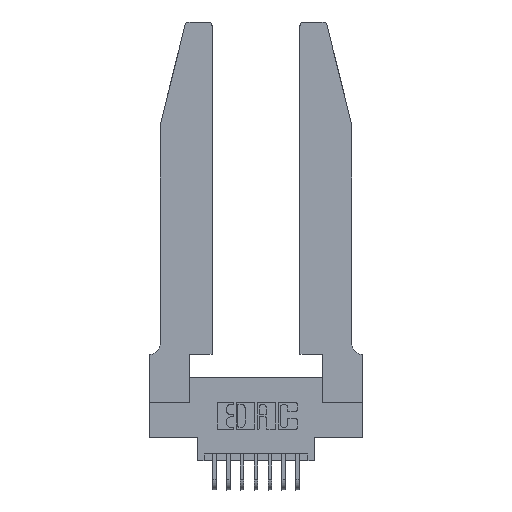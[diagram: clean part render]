
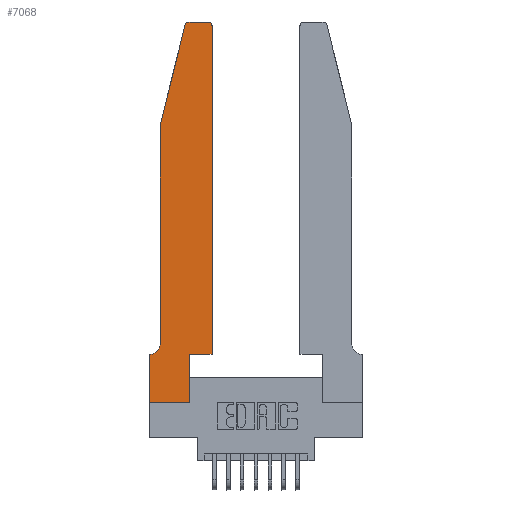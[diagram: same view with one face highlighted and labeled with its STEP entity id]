
A CAD part, top view. The second image highlights one B-rep face of the part: STEP entity #7068.
In plain terms, the highlighted planar face has unit normal (0, 0, 1).
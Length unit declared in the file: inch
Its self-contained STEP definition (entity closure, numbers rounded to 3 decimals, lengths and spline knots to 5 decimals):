
#20 = CARTESIAN_POINT ( 'NONE',  ( 0., 0.35, 0.37 ) ) ;
#129 = VERTEX_POINT ( 'NONE', #14225 ) ;
#232 = VERTEX_POINT ( 'NONE', #20 ) ;
#653 = VECTOR ( 'NONE', #15234, 39.37008 ) ;
#872 = AXIS2_PLACEMENT_3D ( 'NONE', #9520, #1554, #10796 ) ;
#873 = VECTOR ( 'NONE', #11194, 39.37008 ) ;
#876 = VERTEX_POINT ( 'NONE', #8912 ) ;
#995 = VECTOR ( 'NONE', #15243, 39.37008 ) ;
#1045 = VERTEX_POINT ( 'NONE', #2796 ) ;
#1431 = LINE ( 'NONE', #9001, #995 ) ;
#1554 = DIRECTION ( 'NONE',  ( 0., 0., 1. ) ) ;
#1555 = LINE ( 'NONE', #5603, #14964 ) ;
#2014 = CARTESIAN_POINT ( 'NONE',  ( 0.4505, 0.35, 0.37 ) ) ;
#2402 = ORIENTED_EDGE ( 'NONE', *, *, #2558, .T. ) ;
#2558 = EDGE_CURVE ( 'NONE', #129, #6600, #4105, .T. ) ;
#2689 = CARTESIAN_POINT ( 'NONE',  ( 0.2865, 0.35, 0.37 ) ) ;
#2759 = LINE ( 'NONE', #5278, #7181 ) ;
#2796 = CARTESIAN_POINT ( 'NONE',  ( 0.2865, 0., 0.37 ) ) ;
#2841 = VECTOR ( 'NONE', #5559, 39.37008 ) ;
#3032 = VECTOR ( 'NONE', #11817, 39.37008 ) ;
#3412 = AXIS2_PLACEMENT_3D ( 'NONE', #15345, #12888, #5242 ) ;
#4095 = VERTEX_POINT ( 'NONE', #15715 ) ;
#4105 = LINE ( 'NONE', #2014, #873 ) ;
#4113 = CARTESIAN_POINT ( 'NONE',  ( 0.284, 2.72, 0.37 ) ) ;
#4215 = CARTESIAN_POINT ( 'NONE',  ( 0.4505, 0.35, 0.37 ) ) ;
#4342 = VERTEX_POINT ( 'NONE', #11138 ) ;
#5178 = ORIENTED_EDGE ( 'NONE', *, *, #8526, .T. ) ;
#5242 = DIRECTION ( 'NONE',  ( 1., 0., 0. ) ) ;
#5278 = CARTESIAN_POINT ( 'NONE',  ( 0., 0., 0.37 ) ) ;
#5379 = LINE ( 'NONE', #14741, #14745 ) ;
#5454 = DIRECTION ( 'NONE',  ( 1., 0., 0. ) ) ;
#5559 = DIRECTION ( 'NONE',  ( 1., 0., 0. ) ) ;
#5603 = CARTESIAN_POINT ( 'NONE',  ( 0.2605, 2.75, 0.37 ) ) ;
#5798 = EDGE_CURVE ( 'NONE', #10434, #4342, #12495, .T. ) ;
#5986 = ORIENTED_EDGE ( 'NONE', *, *, #7602, .T. ) ;
#6308 = CARTESIAN_POINT ( 'NONE',  ( 0.0755, 2., 0.37 ) ) ;
#6356 = VERTEX_POINT ( 'NONE', #8784 ) ;
#6600 = VERTEX_POINT ( 'NONE', #16669 ) ;
#6928 = DIRECTION ( 'NONE',  ( -1., 0., 0. ) ) ;
#7016 = ORIENTED_EDGE ( 'NONE', *, *, #14909, .T. ) ;
#7060 = FACE_OUTER_BOUND ( 'NONE', #14711, .T. ) ;
#7068 = ADVANCED_FACE ( 'NONE', ( #7060 ), #16506, .T. ) ;
#7117 = CARTESIAN_POINT ( 'NONE',  ( 0.0055, 0.42, 0.37 ) ) ;
#7181 = VECTOR ( 'NONE', #15429, 39.37008 ) ;
#7282 = EDGE_CURVE ( 'NONE', #4342, #876, #10269, .T. ) ;
#7426 = ORIENTED_EDGE ( 'NONE', *, *, #5798, .T. ) ;
#7602 = EDGE_CURVE ( 'NONE', #6600, #14776, #15515, .T. ) ;
#7819 = ORIENTED_EDGE ( 'NONE', *, *, #8131, .T. ) ;
#8131 = EDGE_CURVE ( 'NONE', #876, #232, #5379, .T. ) ;
#8147 = CARTESIAN_POINT ( 'NONE',  ( 0.2865, 0.35, 0.37 ) ) ;
#8221 = ORIENTED_EDGE ( 'NONE', *, *, #10775, .T. ) ;
#8405 = DIRECTION ( 'NONE',  ( -1., 0., 0. ) ) ;
#8526 = EDGE_CURVE ( 'NONE', #1045, #16218, #12956, .T. ) ;
#8631 = ORIENTED_EDGE ( 'NONE', *, *, #13602, .T. ) ;
#8784 = CARTESIAN_POINT ( 'NONE',  ( 0.284, 2.75, 0.37 ) ) ;
#8912 = CARTESIAN_POINT ( 'NONE',  ( 0.0055, 0.35, 0.37 ) ) ;
#9001 = CARTESIAN_POINT ( 'NONE',  ( 0., 0., 0.37 ) ) ;
#9115 = EDGE_CURVE ( 'NONE', #6356, #11110, #15090, .T. ) ;
#9159 = VECTOR ( 'NONE', #14038, 39.37008 ) ;
#9438 = CARTESIAN_POINT ( 'NONE',  ( 0.25487, 2.72718, 0.37 ) ) ;
#9520 = CARTESIAN_POINT ( 'NONE',  ( 0.4205, 2.72, 0.37 ) ) ;
#9709 = EDGE_CURVE ( 'NONE', #4095, #1045, #2759, .T. ) ;
#10269 = CIRCLE ( 'NONE', #10429, 0.07 ) ;
#10429 = AXIS2_PLACEMENT_3D ( 'NONE', #7117, #15914, #8405 ) ;
#10434 = VERTEX_POINT ( 'NONE', #15779 ) ;
#10775 = EDGE_CURVE ( 'NONE', #232, #4095, #1431, .T. ) ;
#10796 = DIRECTION ( 'NONE',  ( 1., 0., 0. ) ) ;
#11110 = VERTEX_POINT ( 'NONE', #9438 ) ;
#11138 = CARTESIAN_POINT ( 'NONE',  ( 0.0755, 0.42, 0.37 ) ) ;
#11194 = DIRECTION ( 'NONE',  ( 0., 1., 0. ) ) ;
#11610 = ORIENTED_EDGE ( 'NONE', *, *, #9709, .T. ) ;
#11817 = DIRECTION ( 'NONE',  ( 0., 1., 0. ) ) ;
#12447 = CARTESIAN_POINT ( 'NONE',  ( 0.4205, 2.75, 0.37 ) ) ;
#12495 = LINE ( 'NONE', #15222, #9159 ) ;
#12888 = DIRECTION ( 'NONE',  ( 0., 0., 1. ) ) ;
#12956 = LINE ( 'NONE', #2689, #3032 ) ;
#12960 = ORIENTED_EDGE ( 'NONE', *, *, #13895, .T. ) ;
#13105 = DIRECTION ( 'NONE',  ( 0., 0., 1. ) ) ;
#13172 = LINE ( 'NONE', #4215, #2841 ) ;
#13513 = DIRECTION ( 'NONE',  ( -1., 0., 0. ) ) ;
#13584 = AXIS2_PLACEMENT_3D ( 'NONE', #4113, #13105, #5454 ) ;
#13602 = EDGE_CURVE ( 'NONE', #16218, #129, #13172, .T. ) ;
#13895 = EDGE_CURVE ( 'NONE', #14776, #6356, #1555, .T. ) ;
#14038 = DIRECTION ( 'NONE',  ( 0., -1., 0. ) ) ;
#14153 = ORIENTED_EDGE ( 'NONE', *, *, #7282, .T. ) ;
#14225 = CARTESIAN_POINT ( 'NONE',  ( 0.4505, 0.35, 0.37 ) ) ;
#14558 = LINE ( 'NONE', #6308, #653 ) ;
#14711 = EDGE_LOOP ( 'NONE', ( #12960, #16622, #7016, #7426, #14153, #7819, #8221, #11610, #5178, #8631, #2402, #5986 ) ) ;
#14741 = CARTESIAN_POINT ( 'NONE',  ( 0.0755, 0.35, 0.37 ) ) ;
#14745 = VECTOR ( 'NONE', #13513, 39.37008 ) ;
#14776 = VERTEX_POINT ( 'NONE', #12447 ) ;
#14909 = EDGE_CURVE ( 'NONE', #11110, #10434, #14558, .T. ) ;
#14964 = VECTOR ( 'NONE', #6928, 39.37008 ) ;
#15090 = CIRCLE ( 'NONE', #13584, 0.03 ) ;
#15222 = CARTESIAN_POINT ( 'NONE',  ( 0.0755, 2., 0.37 ) ) ;
#15234 = DIRECTION ( 'NONE',  ( -0.239, -0.971, 0. ) ) ;
#15243 = DIRECTION ( 'NONE',  ( 0., -1., 0. ) ) ;
#15345 = CARTESIAN_POINT ( 'NONE',  ( 0., 0.35, 0.37 ) ) ;
#15429 = DIRECTION ( 'NONE',  ( 1., 0., 0. ) ) ;
#15515 = CIRCLE ( 'NONE', #872, 0.03 ) ;
#15715 = CARTESIAN_POINT ( 'NONE',  ( 0., 0., 0.37 ) ) ;
#15779 = CARTESIAN_POINT ( 'NONE',  ( 0.0755, 2., 0.37 ) ) ;
#15914 = DIRECTION ( 'NONE',  ( 0., 0., -1. ) ) ;
#16218 = VERTEX_POINT ( 'NONE', #8147 ) ;
#16506 = PLANE ( 'NONE',  #3412 ) ;
#16622 = ORIENTED_EDGE ( 'NONE', *, *, #9115, .T. ) ;
#16669 = CARTESIAN_POINT ( 'NONE',  ( 0.4505, 2.72, 0.37 ) ) ;
